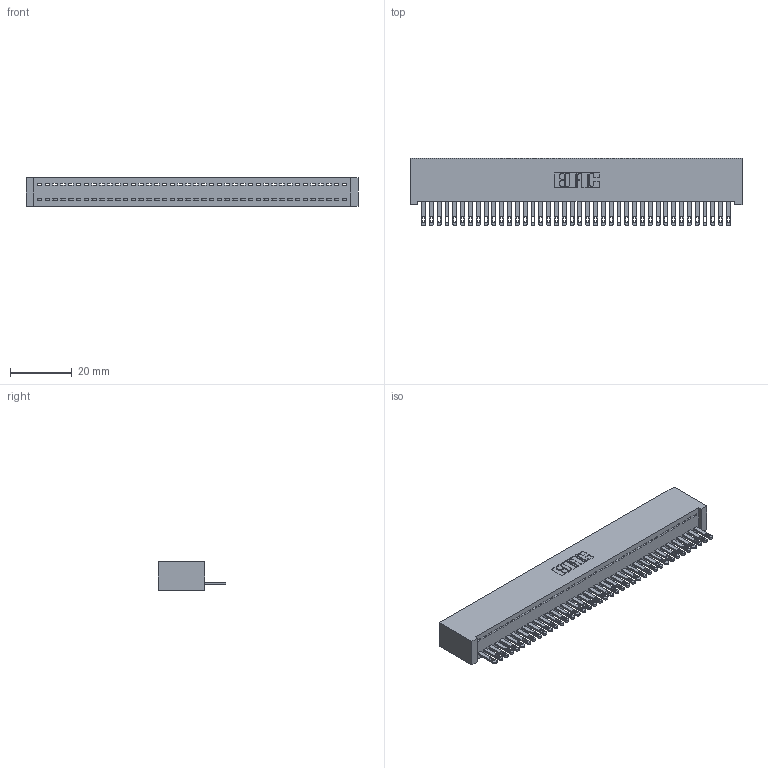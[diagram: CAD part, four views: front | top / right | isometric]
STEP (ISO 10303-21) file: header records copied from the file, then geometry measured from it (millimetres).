
FILE_DESCRIPTION (( 'STEP AP203' ), '1' );
FILE_NAME ('342-040-500-101.STEP', '2019-10-02T15:42:50', ( '' ), ( '' ), 'SwSTEP 2.0', 'SolidWorks 2016', '' );
FILE_SCHEMA (( 'CONFIG_CONTROL_DESIGN' ));
Length unit declared in the file: inch
Products named in the file (3): 342 Part_Lugless; 345-292-001_345-293-100; 342-040-500-101
Assembly tree (41 placements, depth 2):
  342-040-500-101
    342 Part_Lugless
    345-292-001_345-293-100  x40
Bounding box: 107.85 x 21.85 x 9.4 mm (x, y, z)
Volume: 9882.5 mm3; surface area: 14876.7 mm2
Topology: 41 solids, 41 shells, 2262 faces, 6995 edges, 4662 vertices
Faces by surface type: plane 1502, cylinder 760
Entity records: 24233 total; most frequent: CARTESIAN_POINT 4186, ORIENTED_EDGE 4162, DIRECTION 3529, EDGE_CURVE 2081, VECTOR 1957, LINE 1957, VERTEX_POINT 1386, AXIS2_PLACEMENT_3D 786
